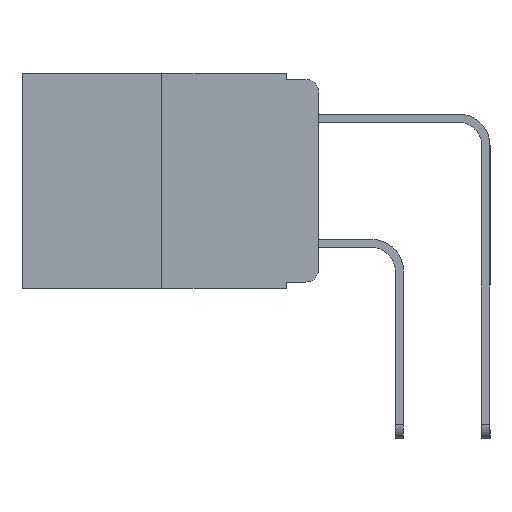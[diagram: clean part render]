
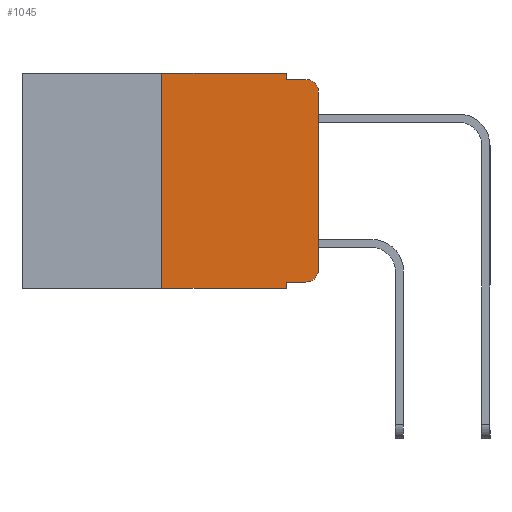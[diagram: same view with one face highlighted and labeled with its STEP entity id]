
A CAD part, left-side view. The second image highlights one B-rep face of the part: STEP entity #1045.
In plain terms, the highlighted planar face has unit normal (-1, 0, 0).
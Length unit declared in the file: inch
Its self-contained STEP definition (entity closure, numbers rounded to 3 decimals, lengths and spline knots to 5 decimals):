
#307 = CARTESIAN_POINT ( 'NONE',  ( 0., 0.051, -0.01 ) ) ;
#308 = VECTOR ( 'NONE', #4129, 39.37008 ) ;
#459 = CARTESIAN_POINT ( 'NONE',  ( 0., 0.02, -0.333 ) ) ;
#664 = ORIENTED_EDGE ( 'NONE', *, *, #1869, .T. ) ;
#680 = LINE ( 'NONE', #5210, #308 ) ;
#769 = AXIS2_PLACEMENT_3D ( 'NONE', #1207, #9745, #7971 ) ;
#839 = EDGE_CURVE ( 'NONE', #1799, #8413, #8523, .T. ) ;
#860 = VERTEX_POINT ( 'NONE', #8448 ) ;
#905 = DIRECTION ( 'NONE',  ( 0., 0., 1. ) ) ;
#976 = CARTESIAN_POINT ( 'NONE',  ( 0., 0.051, -0.333 ) ) ;
#1015 = ORIENTED_EDGE ( 'NONE', *, *, #1696, .F. ) ;
#1045 = ADVANCED_FACE ( 'NONE', ( #3140 ), #12178, .F. ) ;
#1140 = LINE ( 'NONE', #11655, #4866 ) ;
#1207 = CARTESIAN_POINT ( 'NONE',  ( 0., 0.473, 0. ) ) ;
#1608 = ORIENTED_EDGE ( 'NONE', *, *, #2885, .T. ) ;
#1644 = CARTESIAN_POINT ( 'NONE',  ( 0., 0.051, -0.343 ) ) ;
#1696 = EDGE_CURVE ( 'NONE', #11941, #9356, #1140, .T. ) ;
#1701 = VECTOR ( 'NONE', #13127, 39.37008 ) ;
#1799 = VERTEX_POINT ( 'NONE', #459 ) ;
#1869 = EDGE_CURVE ( 'NONE', #1925, #9459, #9725, .T. ) ;
#1886 = ORIENTED_EDGE ( 'NONE', *, *, #8961, .T. ) ;
#1925 = VERTEX_POINT ( 'NONE', #7567 ) ;
#2209 = ORIENTED_EDGE ( 'NONE', *, *, #839, .T. ) ;
#2217 = LINE ( 'NONE', #8280, #12705 ) ;
#2361 = CARTESIAN_POINT ( 'NONE',  ( 0., 0.473, -0.343 ) ) ;
#2373 = EDGE_CURVE ( 'NONE', #9356, #860, #8201, .T. ) ;
#2639 = AXIS2_PLACEMENT_3D ( 'NONE', #4915, #6681, #11604 ) ;
#2673 = CARTESIAN_POINT ( 'NONE',  ( 0., 0.051, 0. ) ) ;
#2762 = EDGE_LOOP ( 'NONE', ( #1886, #3330, #8377, #11861, #1015, #8655, #664, #5323, #1608, #2209 ) ) ;
#2885 = EDGE_CURVE ( 'NONE', #3798, #1799, #2217, .T. ) ;
#3102 = CARTESIAN_POINT ( 'NONE',  ( 0., 0.25, 0. ) ) ;
#3140 = FACE_OUTER_BOUND ( 'NONE', #2762, .T. ) ;
#3294 = CARTESIAN_POINT ( 'NONE',  ( 0., 0.25, 0. ) ) ;
#3330 = ORIENTED_EDGE ( 'NONE', *, *, #6203, .T. ) ;
#3798 = VERTEX_POINT ( 'NONE', #976 ) ;
#3828 = AXIS2_PLACEMENT_3D ( 'NONE', #11283, #5345, #12228 ) ;
#4129 = DIRECTION ( 'NONE',  ( 0., 0., -1. ) ) ;
#4532 = CARTESIAN_POINT ( 'NONE',  ( 0., 0.051, 0. ) ) ;
#4866 = VECTOR ( 'NONE', #8398, 39.37008 ) ;
#4915 = CARTESIAN_POINT ( 'NONE',  ( 0., 0.02, -0.313 ) ) ;
#5210 = CARTESIAN_POINT ( 'NONE',  ( 0., 0.051, 0. ) ) ;
#5323 = ORIENTED_EDGE ( 'NONE', *, *, #9602, .F. ) ;
#5345 = DIRECTION ( 'NONE',  ( -1., 0., 0. ) ) ;
#5399 = DIRECTION ( 'NONE',  ( 0., 0., 1. ) ) ;
#5721 = DIRECTION ( 'NONE',  ( 0., -1., 0. ) ) ;
#6040 = CIRCLE ( 'NONE', #3828, 0.02 ) ;
#6203 = EDGE_CURVE ( 'NONE', #7921, #8267, #6040, .T. ) ;
#6629 = EDGE_CURVE ( 'NONE', #860, #8267, #11874, .T. ) ;
#6681 = DIRECTION ( 'NONE',  ( -1., 0., 0. ) ) ;
#6900 = EDGE_CURVE ( 'NONE', #1925, #11941, #7457, .T. ) ;
#7457 = LINE ( 'NONE', #3294, #12030 ) ;
#7503 = LINE ( 'NONE', #12278, #13253 ) ;
#7567 = CARTESIAN_POINT ( 'NONE',  ( 0., 0.25, -0.343 ) ) ;
#7631 = CARTESIAN_POINT ( 'NONE',  ( 0., 0., -0.03 ) ) ;
#7921 = VERTEX_POINT ( 'NONE', #7631 ) ;
#7971 = DIRECTION ( 'NONE',  ( 0., 0., -1. ) ) ;
#8195 = CARTESIAN_POINT ( 'NONE',  ( 0., 0., -0.313 ) ) ;
#8201 = LINE ( 'NONE', #4532, #11370 ) ;
#8267 = VERTEX_POINT ( 'NONE', #12873 ) ;
#8280 = CARTESIAN_POINT ( 'NONE',  ( 0., 0.051, -0.333 ) ) ;
#8377 = ORIENTED_EDGE ( 'NONE', *, *, #6629, .F. ) ;
#8398 = DIRECTION ( 'NONE',  ( 0., -1., 0. ) ) ;
#8413 = VERTEX_POINT ( 'NONE', #8195 ) ;
#8448 = CARTESIAN_POINT ( 'NONE',  ( 0., 0.051, -0.01 ) ) ;
#8523 = CIRCLE ( 'NONE', #2639, 0.02 ) ;
#8655 = ORIENTED_EDGE ( 'NONE', *, *, #6900, .F. ) ;
#8961 = EDGE_CURVE ( 'NONE', #8413, #7921, #7503, .T. ) ;
#9307 = VECTOR ( 'NONE', #10754, 39.37008 ) ;
#9356 = VERTEX_POINT ( 'NONE', #2673 ) ;
#9459 = VERTEX_POINT ( 'NONE', #1644 ) ;
#9602 = EDGE_CURVE ( 'NONE', #3798, #9459, #680, .T. ) ;
#9725 = LINE ( 'NONE', #2361, #1701 ) ;
#9745 = DIRECTION ( 'NONE',  ( 1., 0., 0. ) ) ;
#10157 = DIRECTION ( 'NONE',  ( 0., 0., -1. ) ) ;
#10754 = DIRECTION ( 'NONE',  ( 0., -1., 0. ) ) ;
#11283 = CARTESIAN_POINT ( 'NONE',  ( 0., 0.02, -0.03 ) ) ;
#11370 = VECTOR ( 'NONE', #10157, 39.37008 ) ;
#11604 = DIRECTION ( 'NONE',  ( 0., 0., -1. ) ) ;
#11655 = CARTESIAN_POINT ( 'NONE',  ( 0., 0.473, 0. ) ) ;
#11861 = ORIENTED_EDGE ( 'NONE', *, *, #2373, .F. ) ;
#11874 = LINE ( 'NONE', #307, #9307 ) ;
#11941 = VERTEX_POINT ( 'NONE', #3102 ) ;
#12030 = VECTOR ( 'NONE', #905, 39.37008 ) ;
#12178 = PLANE ( 'NONE',  #769 ) ;
#12228 = DIRECTION ( 'NONE',  ( 0., 0., -1. ) ) ;
#12278 = CARTESIAN_POINT ( 'NONE',  ( 0., 0., 0. ) ) ;
#12705 = VECTOR ( 'NONE', #5721, 39.37008 ) ;
#12873 = CARTESIAN_POINT ( 'NONE',  ( 0., 0.02, -0.01 ) ) ;
#13127 = DIRECTION ( 'NONE',  ( 0., -1., 0. ) ) ;
#13253 = VECTOR ( 'NONE', #5399, 39.37008 ) ;
